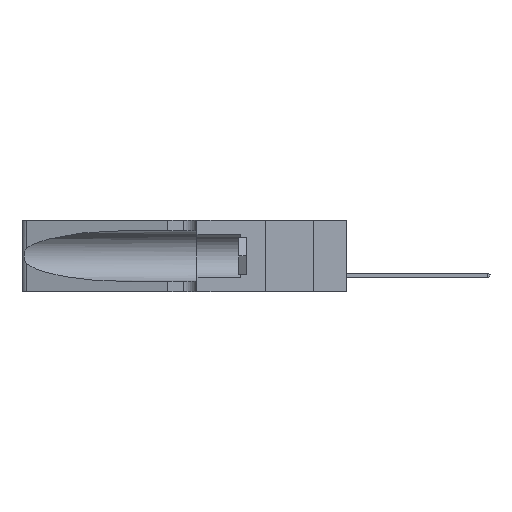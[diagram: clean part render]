
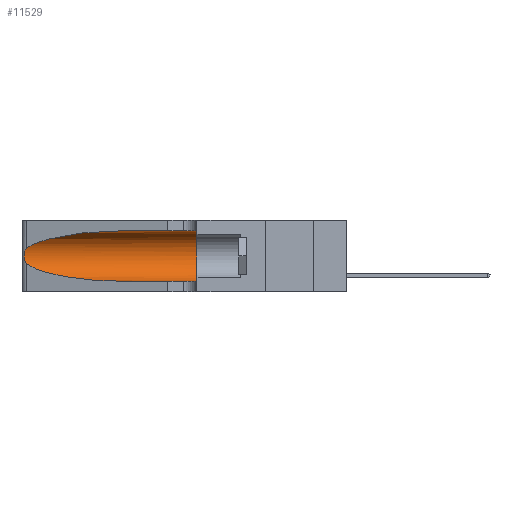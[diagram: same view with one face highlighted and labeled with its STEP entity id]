
A CAD part, left-side view. The second image highlights one B-rep face of the part: STEP entity #11529.
In plain terms, the highlighted cylindrical face has radius 3.308 mm (diameter 6.617 mm), a partial arc.
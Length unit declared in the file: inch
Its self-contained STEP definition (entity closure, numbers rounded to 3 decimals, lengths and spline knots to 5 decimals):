
#562 = CARTESIAN_POINT ( 'NONE',  ( 0.1305, 0.72297, 0.31525 ) ) ;
#865 =( BOUNDED_CURVE ( )  B_SPLINE_CURVE ( 3, ( #2210, #16271, #26828, #29497 ),
 .UNSPECIFIED., .F., .T. ) 
 B_SPLINE_CURVE_WITH_KNOTS ( ( 4, 4 ),
 ( 1.5708, 2.84003 ),
 .UNSPECIFIED. ) 
 CURVE ( )  GEOMETRIC_REPRESENTATION_ITEM ( )  RATIONAL_B_SPLINE_CURVE ( ( 1., 0.87, 0.87, 1. ) ) 
 REPRESENTATION_ITEM ( '' )  );
#1283 = CARTESIAN_POINT ( 'NONE',  ( 0.25487, 1.22718, 0.14631 ) ) ;
#1919 = VERTEX_POINT ( 'NONE', #15783 ) ;
#2210 = CARTESIAN_POINT ( 'NONE',  ( 0.1305, 0.72297, 0.31525 ) ) ;
#2659 = CARTESIAN_POINT ( 'NONE',  ( 0.1305, 1.61858, 0.31525 ) ) ;
#4450 = VERTEX_POINT ( 'NONE', #31641 ) ;
#6265 = ORIENTED_EDGE ( 'NONE', *, *, #29558, .F. ) ;
#7740 = CARTESIAN_POINT ( 'NONE',  ( 0.25787, 1.23484, 0.2124 ) ) ;
#8203 = VERTEX_POINT ( 'NONE', #14055 ) ;
#8477 = EDGE_CURVE ( 'NONE', #4450, #37537, #29703, .T. ) ;
#8948 = AXIS2_PLACEMENT_3D ( 'NONE', #41111, #41261, #21977 ) ;
#9273 = CYLINDRICAL_SURFACE ( 'NONE', #8948, 0.13025 ) ;
#10955 = CARTESIAN_POINT ( 'NONE',  ( 0.26075, 1.23896, 0.19203 ) ) ;
#10958 =( BOUNDED_CURVE ( )  B_SPLINE_CURVE ( 3, ( #21042, #18081, #24184, #40608 ),
 .UNSPECIFIED., .F., .T. ) 
 B_SPLINE_CURVE_WITH_KNOTS ( ( 4, 4 ),
 ( 3.44316, 4.71239 ),
 .UNSPECIFIED. ) 
 CURVE ( )  GEOMETRIC_REPRESENTATION_ITEM ( )  RATIONAL_B_SPLINE_CURVE ( ( 1., 0.87, 0.87, 1. ) ) 
 REPRESENTATION_ITEM ( '' )  );
#11529 = ADVANCED_FACE ( 'NONE', ( #17805 ), #9273, .F. ) ;
#11640 = ORIENTED_EDGE ( 'NONE', *, *, #8477, .F. ) ;
#11924 = CARTESIAN_POINT ( 'NONE',  ( 0.25487, 1.22718, 0.22369 ) ) ;
#13917 = CARTESIAN_POINT ( 'NONE',  ( 0.25555, 1.22994, 0.2215 ) ) ;
#14055 = CARTESIAN_POINT ( 'NONE',  ( 0.1305, 0.72297, 0.05475 ) ) ;
#14186 = EDGE_CURVE ( 'NONE', #30165, #19357, #865, .T. ) ;
#14210 = CARTESIAN_POINT ( 'NONE',  ( 0.26075, 1.23896, 0.178 ) ) ;
#14415 = ORIENTED_EDGE ( 'NONE', *, *, #37944, .T. ) ;
#14647 = EDGE_CURVE ( 'NONE', #19357, #1919, #21591, .T. ) ;
#15084 = AXIS2_PLACEMENT_3D ( 'NONE', #24970, #41116, #21840 ) ;
#15783 = CARTESIAN_POINT ( 'NONE',  ( 0.25487, 1.22718, 0.14631 ) ) ;
#16216 = ORIENTED_EDGE ( 'NONE', *, *, #14186, .T. ) ;
#16271 = CARTESIAN_POINT ( 'NONE',  ( 0.18966, 0.96281, 0.31525 ) ) ;
#16285 = CARTESIAN_POINT ( 'NONE',  ( 0.25789, 1.23486, 0.15765 ) ) ;
#16524 = ORIENTED_EDGE ( 'NONE', *, *, #18503, .T. ) ;
#17166 = CARTESIAN_POINT ( 'NONE',  ( 0.26018, 1.23835, 0.19895 ) ) ;
#17805 = FACE_OUTER_BOUND ( 'NONE', #25963, .T. ) ;
#18081 = CARTESIAN_POINT ( 'NONE',  ( 0.2373, 1.15595, 0.08982 ) ) ;
#18503 = EDGE_CURVE ( 'NONE', #8203, #37537, #37785, .T. ) ;
#19357 = VERTEX_POINT ( 'NONE', #11924 ) ;
#21042 = CARTESIAN_POINT ( 'NONE',  ( 0.25487, 1.22718, 0.14631 ) ) ;
#21591 = B_SPLINE_CURVE_WITH_KNOTS ( 'NONE', 3,
 ( #27070, #13917, #36465, #7740, #30295, #17166, #10955, #14210, #25251, #28040, #16285, #40322, #29724, #1283 ),
 .UNSPECIFIED., .F., .F.,
 ( 4, 2, 2, 2, 2, 2, 4 ),
 ( 0., 0.00027, 0.00053, 0.00107, 0.0016, 0.00187, 0.00214 ),
 .UNSPECIFIED. ) ;
#21840 = DIRECTION ( 'NONE',  ( 0., 0., 1. ) ) ;
#21977 = DIRECTION ( 'NONE',  ( 0., 0., -1. ) ) ;
#24034 = VECTOR ( 'NONE', #41393, 39.37008 ) ;
#24184 = CARTESIAN_POINT ( 'NONE',  ( 0.18966, 0.96281, 0.05475 ) ) ;
#24970 = CARTESIAN_POINT ( 'NONE',  ( 0.1305, 0.35, 0.185 ) ) ;
#25251 = CARTESIAN_POINT ( 'NONE',  ( 0.26017, 1.23833, 0.17102 ) ) ;
#25636 = CARTESIAN_POINT ( 'NONE',  ( 0.1305, 0.35, 0.05475 ) ) ;
#25963 = EDGE_LOOP ( 'NONE', ( #16216, #28742, #14415, #16524, #11640, #6265 ) ) ;
#26828 = CARTESIAN_POINT ( 'NONE',  ( 0.2373, 1.15595, 0.28018 ) ) ;
#27070 = CARTESIAN_POINT ( 'NONE',  ( 0.25487, 1.22718, 0.22369 ) ) ;
#28040 = CARTESIAN_POINT ( 'NONE',  ( 0.25856, 1.23593, 0.16098 ) ) ;
#28742 = ORIENTED_EDGE ( 'NONE', *, *, #14647, .T. ) ;
#29497 = CARTESIAN_POINT ( 'NONE',  ( 0.25487, 1.22718, 0.22369 ) ) ;
#29558 = EDGE_CURVE ( 'NONE', #30165, #4450, #39620, .T. ) ;
#29703 = CIRCLE ( 'NONE', #15084, 0.13025 ) ;
#29724 = CARTESIAN_POINT ( 'NONE',  ( 0.25555, 1.22993, 0.14849 ) ) ;
#30165 = VERTEX_POINT ( 'NONE', #562 ) ;
#30295 = CARTESIAN_POINT ( 'NONE',  ( 0.25854, 1.2359, 0.20912 ) ) ;
#30728 = VECTOR ( 'NONE', #31539, 39.37008 ) ;
#31539 = DIRECTION ( 'NONE',  ( 0., -1., 0. ) ) ;
#31641 = CARTESIAN_POINT ( 'NONE',  ( 0.1305, 0.35, 0.31525 ) ) ;
#34172 = CARTESIAN_POINT ( 'NONE',  ( 0.1305, 1.61858, 0.05475 ) ) ;
#36465 = CARTESIAN_POINT ( 'NONE',  ( 0.25639, 1.23184, 0.21858 ) ) ;
#37537 = VERTEX_POINT ( 'NONE', #25636 ) ;
#37785 = LINE ( 'NONE', #34172, #30728 ) ;
#37944 = EDGE_CURVE ( 'NONE', #1919, #8203, #10958, .T. ) ;
#39620 = LINE ( 'NONE', #2659, #24034 ) ;
#40322 = CARTESIAN_POINT ( 'NONE',  ( 0.25639, 1.23186, 0.15144 ) ) ;
#40608 = CARTESIAN_POINT ( 'NONE',  ( 0.1305, 0.72297, 0.05475 ) ) ;
#41111 = CARTESIAN_POINT ( 'NONE',  ( 0.1305, 1.61858, 0.185 ) ) ;
#41116 = DIRECTION ( 'NONE',  ( 0., 1., 0. ) ) ;
#41261 = DIRECTION ( 'NONE',  ( 0., -1., 0. ) ) ;
#41393 = DIRECTION ( 'NONE',  ( 0., -1., 0. ) ) ;
